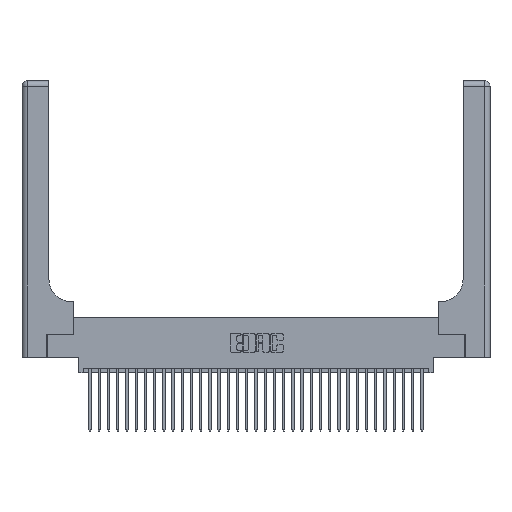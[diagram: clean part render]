
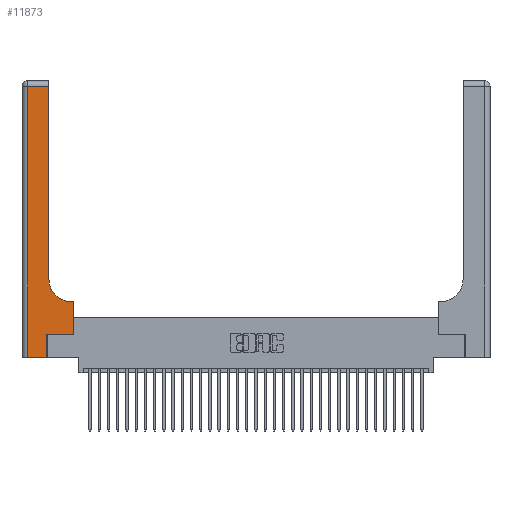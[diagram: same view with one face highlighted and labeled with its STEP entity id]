
A CAD part, top view. The second image highlights one B-rep face of the part: STEP entity #11873.
In plain terms, the highlighted planar face has unit normal (0, 0, 1).
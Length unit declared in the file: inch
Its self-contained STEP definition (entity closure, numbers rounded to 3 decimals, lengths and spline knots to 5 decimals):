
#62 = AXIS2_PLACEMENT_3D ( 'NONE', #15382, #34230, #18110 ) ;
#267 = VERTEX_POINT ( 'NONE', #17767 ) ;
#1764 = DIRECTION ( 'NONE',  ( 0., 1., 0. ) ) ;
#2342 = CARTESIAN_POINT ( 'NONE',  ( 0.269, 0.25, 0.37 ) ) ;
#2445 = CARTESIAN_POINT ( 'NONE',  ( 0.269, 0., 0.37 ) ) ;
#2623 = VERTEX_POINT ( 'NONE', #31348 ) ;
#2626 = PLANE ( 'NONE',  #29474 ) ;
#3018 = CARTESIAN_POINT ( 'NONE',  ( 0.2915, 0.6, 0.37 ) ) ;
#3553 = CARTESIAN_POINT ( 'NONE',  ( 0.06, 3., 0.37 ) ) ;
#3585 = EDGE_CURVE ( 'NONE', #2623, #33721, #33920, .T. ) ;
#4652 = VERTEX_POINT ( 'NONE', #18919 ) ;
#4887 = VECTOR ( 'NONE', #29409, 39.37008 ) ;
#5475 = EDGE_CURVE ( 'NONE', #7410, #2623, #15217, .T. ) ;
#5726 = LINE ( 'NONE', #2342, #4887 ) ;
#6776 = CARTESIAN_POINT ( 'NONE',  ( 0.5585, 0.25, 0.37 ) ) ;
#6825 = ORIENTED_EDGE ( 'NONE', *, *, #12302, .T. ) ;
#7134 = VECTOR ( 'NONE', #22734, 39.37008 ) ;
#7396 = ORIENTED_EDGE ( 'NONE', *, *, #29861, .T. ) ;
#7410 = VERTEX_POINT ( 'NONE', #33435 ) ;
#7799 = ORIENTED_EDGE ( 'NONE', *, *, #19959, .T. ) ;
#9160 = VECTOR ( 'NONE', #10978, 39.37008 ) ;
#10764 = LINE ( 'NONE', #20692, #34391 ) ;
#10841 = DIRECTION ( 'NONE',  ( 0., 0., -1. ) ) ;
#10925 = ORIENTED_EDGE ( 'NONE', *, *, #11417, .T. ) ;
#10978 = DIRECTION ( 'NONE',  ( 0., 1., 0. ) ) ;
#11417 = EDGE_CURVE ( 'NONE', #267, #14418, #21188, .T. ) ;
#11873 = ADVANCED_FACE ( 'NONE', ( #20552 ), #2626, .F. ) ;
#12302 = EDGE_CURVE ( 'NONE', #33721, #17751, #21377, .T. ) ;
#14418 = VERTEX_POINT ( 'NONE', #24405 ) ;
#15217 = LINE ( 'NONE', #3553, #7134 ) ;
#15285 = CARTESIAN_POINT ( 'NONE',  ( 0.269, 0.25, 0.37 ) ) ;
#15382 = CARTESIAN_POINT ( 'NONE',  ( 0.5415, 0.85, 0.37 ) ) ;
#15722 = ORIENTED_EDGE ( 'NONE', *, *, #17966, .T. ) ;
#15765 = DIRECTION ( 'NONE',  ( 0., 1., 0. ) ) ;
#16270 = ORIENTED_EDGE ( 'NONE', *, *, #23000, .T. ) ;
#16325 = CARTESIAN_POINT ( 'NONE',  ( 0.5585, 0.25, 0.37 ) ) ;
#17305 = ORIENTED_EDGE ( 'NONE', *, *, #31638, .T. ) ;
#17353 = ORIENTED_EDGE ( 'NONE', *, *, #3585, .T. ) ;
#17751 = VERTEX_POINT ( 'NONE', #15285 ) ;
#17767 = CARTESIAN_POINT ( 'NONE',  ( 0.5585, 0.6, 0.37 ) ) ;
#17966 = EDGE_CURVE ( 'NONE', #28896, #267, #29823, .T. ) ;
#18110 = DIRECTION ( 'NONE',  ( 1., 0., 0. ) ) ;
#18919 = CARTESIAN_POINT ( 'NONE',  ( 0.2915, 0.85, 0.37 ) ) ;
#19048 = VERTEX_POINT ( 'NONE', #33795 ) ;
#19440 = DIRECTION ( 'NONE',  ( 1., 0., 0. ) ) ;
#19959 = EDGE_CURVE ( 'NONE', #19048, #7410, #10764, .T. ) ;
#20332 = VECTOR ( 'NONE', #30065, 39.37008 ) ;
#20552 = FACE_OUTER_BOUND ( 'NONE', #21048, .T. ) ;
#20692 = CARTESIAN_POINT ( 'NONE',  ( 0., 2.94, 0.37 ) ) ;
#21048 = EDGE_LOOP ( 'NONE', ( #7396, #7799, #30506, #17353, #6825, #17305, #15722, #10925, #16270 ) ) ;
#21188 = LINE ( 'NONE', #3018, #20332 ) ;
#21377 = LINE ( 'NONE', #34177, #29356 ) ;
#22734 = DIRECTION ( 'NONE',  ( 0., -1., 0. ) ) ;
#23000 = EDGE_CURVE ( 'NONE', #14418, #4652, #24880, .T. ) ;
#23761 = CARTESIAN_POINT ( 'NONE',  ( 0.2915, 3., 0.37 ) ) ;
#24405 = CARTESIAN_POINT ( 'NONE',  ( 0.5415, 0.6, 0.37 ) ) ;
#24880 = CIRCLE ( 'NONE', #62, 0.25 ) ;
#25985 = VECTOR ( 'NONE', #15765, 39.37008 ) ;
#26761 = VECTOR ( 'NONE', #19440, 39.37008 ) ;
#26840 = LINE ( 'NONE', #23761, #25985 ) ;
#27008 = CARTESIAN_POINT ( 'NONE',  ( 0., 3., 0.37 ) ) ;
#28896 = VERTEX_POINT ( 'NONE', #6776 ) ;
#29356 = VECTOR ( 'NONE', #1764, 39.37008 ) ;
#29409 = DIRECTION ( 'NONE',  ( 1., 0., 0. ) ) ;
#29474 = AXIS2_PLACEMENT_3D ( 'NONE', #27008, #10841, #29689 ) ;
#29689 = DIRECTION ( 'NONE',  ( -1., 0., 0. ) ) ;
#29823 = LINE ( 'NONE', #16325, #9160 ) ;
#29861 = EDGE_CURVE ( 'NONE', #4652, #19048, #26840, .T. ) ;
#30065 = DIRECTION ( 'NONE',  ( -1., 0., 0. ) ) ;
#30117 = CARTESIAN_POINT ( 'NONE',  ( 0., 0., 0.37 ) ) ;
#30506 = ORIENTED_EDGE ( 'NONE', *, *, #5475, .T. ) ;
#31348 = CARTESIAN_POINT ( 'NONE',  ( 0.06, 0., 0.37 ) ) ;
#31377 = DIRECTION ( 'NONE',  ( -1., 0., 0. ) ) ;
#31638 = EDGE_CURVE ( 'NONE', #17751, #28896, #5726, .T. ) ;
#33435 = CARTESIAN_POINT ( 'NONE',  ( 0.06, 2.94, 0.37 ) ) ;
#33721 = VERTEX_POINT ( 'NONE', #2445 ) ;
#33795 = CARTESIAN_POINT ( 'NONE',  ( 0.2915, 2.94, 0.37 ) ) ;
#33920 = LINE ( 'NONE', #30117, #26761 ) ;
#34177 = CARTESIAN_POINT ( 'NONE',  ( 0.269, 0., 0.37 ) ) ;
#34230 = DIRECTION ( 'NONE',  ( 0., 0., -1. ) ) ;
#34391 = VECTOR ( 'NONE', #31377, 39.37008 ) ;
